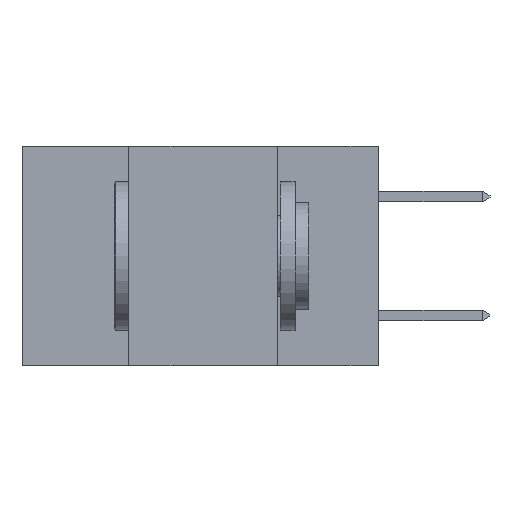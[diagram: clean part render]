
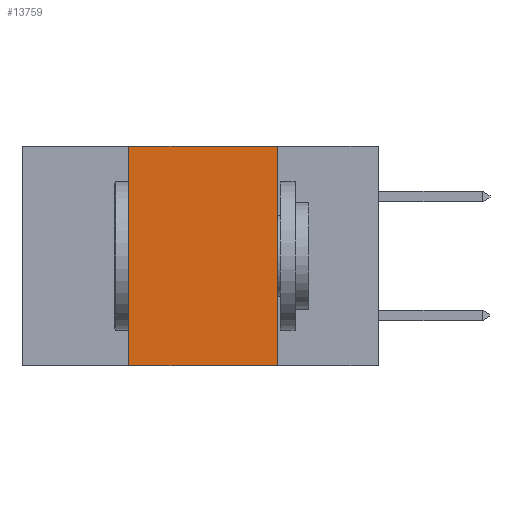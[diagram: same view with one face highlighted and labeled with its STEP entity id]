
A CAD part, left-side view. The second image highlights one B-rep face of the part: STEP entity #13759.
In plain terms, the highlighted planar face has unit normal (-1, 0, 0).
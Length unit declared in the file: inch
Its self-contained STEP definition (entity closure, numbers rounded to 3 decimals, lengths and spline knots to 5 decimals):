
#171 = DIRECTION ( 'NONE',  ( 0., -1., 0. ) ) ;
#3485 = ORIENTED_EDGE ( 'NONE', *, *, #18357, .T. ) ;
#5782 = CARTESIAN_POINT ( 'NONE',  ( 0., 0.42, -0.37 ) ) ;
#5829 = VERTEX_POINT ( 'NONE', #23745 ) ;
#7598 = EDGE_CURVE ( 'NONE', #11773, #5829, #23731, .T. ) ;
#7761 = VECTOR ( 'NONE', #28200, 39.37008 ) ;
#10863 = CARTESIAN_POINT ( 'NONE',  ( 0., 0.17, 0. ) ) ;
#11050 = LINE ( 'NONE', #11419, #11726 ) ;
#11419 = CARTESIAN_POINT ( 'NONE',  ( 0., 0.6, 0. ) ) ;
#11509 = DIRECTION ( 'NONE',  ( 0., -1., 0. ) ) ;
#11726 = VECTOR ( 'NONE', #11509, 39.37008 ) ;
#11773 = VERTEX_POINT ( 'NONE', #26707 ) ;
#11949 = VECTOR ( 'NONE', #20805, 39.37008 ) ;
#12051 = DIRECTION ( 'NONE',  ( 1., 0., 0. ) ) ;
#12499 = VECTOR ( 'NONE', #171, 39.37008 ) ;
#13031 = ORIENTED_EDGE ( 'NONE', *, *, #21566, .F. ) ;
#13347 = CARTESIAN_POINT ( 'NONE',  ( 0., 0.6, -0.37 ) ) ;
#13759 = ADVANCED_FACE ( 'NONE', ( #27773 ), #25047, .F. ) ;
#14118 = CARTESIAN_POINT ( 'NONE',  ( 0., 0.6, 0. ) ) ;
#14218 = CARTESIAN_POINT ( 'NONE',  ( 0., 0.42, 0. ) ) ;
#18357 = EDGE_CURVE ( 'NONE', #26580, #5829, #23370, .T. ) ;
#19691 = EDGE_CURVE ( 'NONE', #24627, #11773, #11050, .T. ) ;
#20044 = AXIS2_PLACEMENT_3D ( 'NONE', #14118, #12051, #27268 ) ;
#20805 = DIRECTION ( 'NONE',  ( 0., 0., 1. ) ) ;
#20892 = ORIENTED_EDGE ( 'NONE', *, *, #19691, .F. ) ;
#21216 = ORIENTED_EDGE ( 'NONE', *, *, #7598, .F. ) ;
#21566 = EDGE_CURVE ( 'NONE', #26580, #24627, #24169, .T. ) ;
#23079 = CARTESIAN_POINT ( 'NONE',  ( 0., 0.42, 0. ) ) ;
#23111 = EDGE_LOOP ( 'NONE', ( #21216, #20892, #13031, #3485 ) ) ;
#23370 = LINE ( 'NONE', #13347, #12499 ) ;
#23731 = LINE ( 'NONE', #10863, #7761 ) ;
#23745 = CARTESIAN_POINT ( 'NONE',  ( 0., 0.17, -0.37 ) ) ;
#24169 = LINE ( 'NONE', #14218, #11949 ) ;
#24627 = VERTEX_POINT ( 'NONE', #23079 ) ;
#25047 = PLANE ( 'NONE',  #20044 ) ;
#26580 = VERTEX_POINT ( 'NONE', #5782 ) ;
#26707 = CARTESIAN_POINT ( 'NONE',  ( 0., 0.17, 0. ) ) ;
#27268 = DIRECTION ( 'NONE',  ( 0., 0., -1. ) ) ;
#27773 = FACE_OUTER_BOUND ( 'NONE', #23111, .T. ) ;
#28200 = DIRECTION ( 'NONE',  ( 0., 0., -1. ) ) ;
